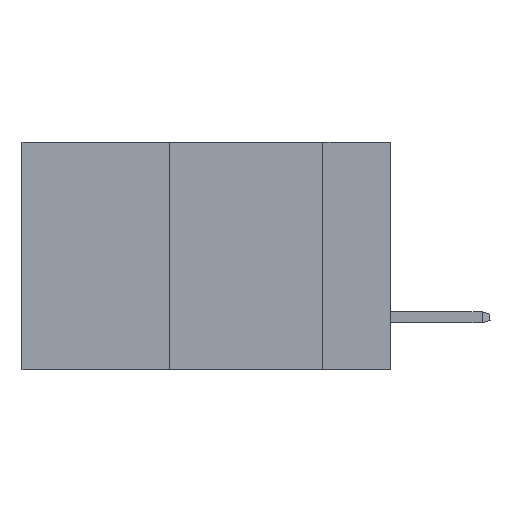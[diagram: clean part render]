
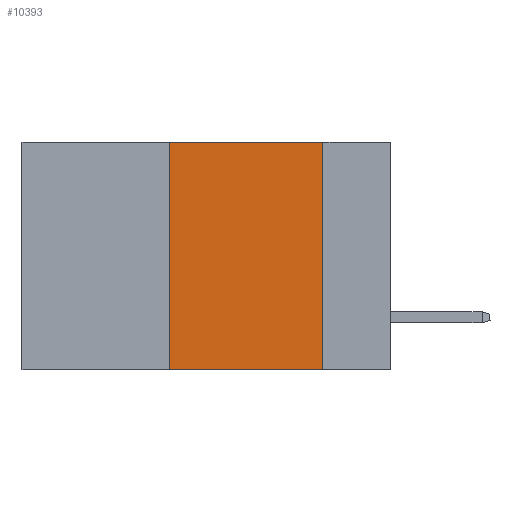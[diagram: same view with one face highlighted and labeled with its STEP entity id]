
A CAD part, left-side view. The second image highlights one B-rep face of the part: STEP entity #10393.
In plain terms, the highlighted planar face has unit normal (-1, 0, 0).
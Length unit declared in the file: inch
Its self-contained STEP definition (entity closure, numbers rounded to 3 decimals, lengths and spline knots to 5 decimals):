
#1696 = DIRECTION ( 'NONE',  ( 0., 0., -1. ) ) ;
#1818 = EDGE_CURVE ( 'NONE', #23364, #16943, #9949, .T. ) ;
#5198 = DIRECTION ( 'NONE',  ( 0., -1., 0. ) ) ;
#5795 = ORIENTED_EDGE ( 'NONE', *, *, #16114, .F. ) ;
#6687 = DIRECTION ( 'NONE',  ( 0., 0., 1. ) ) ;
#7140 = CARTESIAN_POINT ( 'NONE',  ( 0., 0.6, -0.37 ) ) ;
#7179 = PLANE ( 'NONE',  #15109 ) ;
#7326 = CARTESIAN_POINT ( 'NONE',  ( 0., 0.11, 0. ) ) ;
#8733 = VECTOR ( 'NONE', #8870, 39.37008 ) ;
#8870 = DIRECTION ( 'NONE',  ( 0., -1., 0. ) ) ;
#9132 = DIRECTION ( 'NONE',  ( 1., 0., 0. ) ) ;
#9949 = LINE ( 'NONE', #18090, #8733 ) ;
#10393 = ADVANCED_FACE ( 'NONE', ( #16898 ), #7179, .F. ) ;
#11218 = CARTESIAN_POINT ( 'NONE',  ( 0., 0.11, -0.37 ) ) ;
#11343 = EDGE_CURVE ( 'NONE', #16763, #23364, #11714, .T. ) ;
#11714 = LINE ( 'NONE', #18280, #23210 ) ;
#11886 = CARTESIAN_POINT ( 'NONE',  ( 0., 0.36, -0.37 ) ) ;
#12538 = VECTOR ( 'NONE', #15906, 39.37008 ) ;
#12981 = LINE ( 'NONE', #21480, #12538 ) ;
#13698 = ORIENTED_EDGE ( 'NONE', *, *, #1818, .F. ) ;
#14015 = EDGE_LOOP ( 'NONE', ( #5795, #13698, #15489, #21905 ) ) ;
#14538 = VERTEX_POINT ( 'NONE', #11218 ) ;
#15109 = AXIS2_PLACEMENT_3D ( 'NONE', #20722, #9132, #1696 ) ;
#15489 = ORIENTED_EDGE ( 'NONE', *, *, #11343, .F. ) ;
#15906 = DIRECTION ( 'NONE',  ( 0., 0., -1. ) ) ;
#16114 = EDGE_CURVE ( 'NONE', #16943, #14538, #12981, .T. ) ;
#16763 = VERTEX_POINT ( 'NONE', #11886 ) ;
#16898 = FACE_OUTER_BOUND ( 'NONE', #14015, .T. ) ;
#16943 = VERTEX_POINT ( 'NONE', #7326 ) ;
#18090 = CARTESIAN_POINT ( 'NONE',  ( 0., 0.6, 0. ) ) ;
#18280 = CARTESIAN_POINT ( 'NONE',  ( 0., 0.36, 0. ) ) ;
#18763 = LINE ( 'NONE', #7140, #21802 ) ;
#20722 = CARTESIAN_POINT ( 'NONE',  ( 0., 0.6, 0. ) ) ;
#21480 = CARTESIAN_POINT ( 'NONE',  ( 0., 0.11, 0. ) ) ;
#21802 = VECTOR ( 'NONE', #5198, 39.37008 ) ;
#21905 = ORIENTED_EDGE ( 'NONE', *, *, #24785, .T. ) ;
#22593 = CARTESIAN_POINT ( 'NONE',  ( 0., 0.36, 0. ) ) ;
#23210 = VECTOR ( 'NONE', #6687, 39.37008 ) ;
#23364 = VERTEX_POINT ( 'NONE', #22593 ) ;
#24785 = EDGE_CURVE ( 'NONE', #16763, #14538, #18763, .T. ) ;
